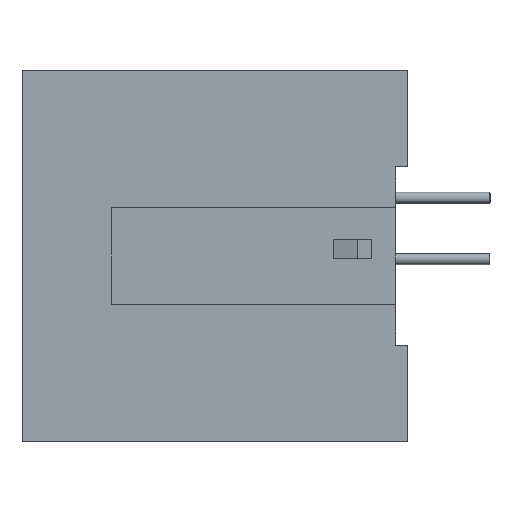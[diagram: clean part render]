
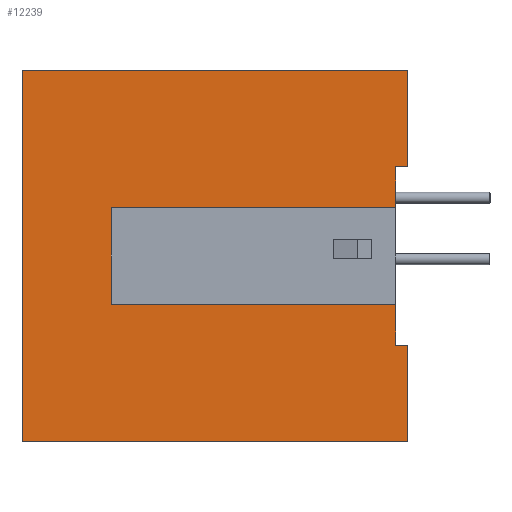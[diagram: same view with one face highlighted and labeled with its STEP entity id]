
A CAD part, left-side view. The second image highlights one B-rep face of the part: STEP entity #12239.
In plain terms, the highlighted planar face has unit normal (-1, 0, 0).
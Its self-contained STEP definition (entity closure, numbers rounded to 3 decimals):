
#409 = EDGE_CURVE ( 'NONE', #6827, #12593, #609, .T. ) ;
#457 = DIRECTION ( 'NONE',  ( 0., 0., 1. ) ) ;
#609 = LINE ( 'NONE', #684, #3271 ) ;
#684 = CARTESIAN_POINT ( 'NONE',  ( -27.5, 4., 0. ) ) ;
#745 = LINE ( 'NONE', #11575, #10384 ) ;
#837 = LINE ( 'NONE', #3326, #9380 ) ;
#955 = ORIENTED_EDGE ( 'NONE', *, *, #2630, .T. ) ;
#1096 = LINE ( 'NONE', #13087, #2777 ) ;
#1269 = CARTESIAN_POINT ( 'NONE',  ( -27.5, -8.3, 7.7 ) ) ;
#1413 = LINE ( 'NONE', #6178, #6186 ) ;
#1547 = LINE ( 'NONE', #4185, #4144 ) ;
#1643 = CARTESIAN_POINT ( 'NONE',  ( -27.5, -0.3, 1.8 ) ) ;
#1660 = VECTOR ( 'NONE', #3234, 1000. ) ;
#1877 = LINE ( 'NONE', #1643, #12169 ) ;
#2078 = ORIENTED_EDGE ( 'NONE', *, *, #5729, .F. ) ;
#2206 = CARTESIAN_POINT ( 'NONE',  ( -27.5, -7.8, 1.8 ) ) ;
#2349 = CARTESIAN_POINT ( 'NONE',  ( -27.5, 4., 1.8 ) ) ;
#2397 = VERTEX_POINT ( 'NONE', #2206 ) ;
#2450 = VERTEX_POINT ( 'NONE', #8057 ) ;
#2509 = CARTESIAN_POINT ( 'NONE',  ( -27.5, -8.3, -3.7 ) ) ;
#2519 = CARTESIAN_POINT ( 'NONE',  ( -27.5, -0.3, -7.7 ) ) ;
#2630 = EDGE_CURVE ( 'NONE', #14668, #4845, #1413, .T. ) ;
#2739 = ORIENTED_EDGE ( 'NONE', *, *, #7478, .F. ) ;
#2777 = VECTOR ( 'NONE', #5856, 1000. ) ;
#2883 = LINE ( 'NONE', #2519, #10856 ) ;
#3023 = VECTOR ( 'NONE', #14597, 1000. ) ;
#3026 = ORIENTED_EDGE ( 'NONE', *, *, #3966, .F. ) ;
#3234 = DIRECTION ( 'NONE',  ( 0., -1., 0. ) ) ;
#3271 = VECTOR ( 'NONE', #13538, 1000. ) ;
#3326 = CARTESIAN_POINT ( 'NONE',  ( -27.5, -0.3, 3.7 ) ) ;
#3514 = VECTOR ( 'NONE', #11791, 1000. ) ;
#3703 = VERTEX_POINT ( 'NONE', #2509 ) ;
#3966 = EDGE_CURVE ( 'NONE', #5069, #11071, #1096, .T. ) ;
#4144 = VECTOR ( 'NONE', #7702, 1000. ) ;
#4185 = CARTESIAN_POINT ( 'NONE',  ( -27.5, -0.3, -1.8 ) ) ;
#4594 = FACE_OUTER_BOUND ( 'NONE', #12394, .T. ) ;
#4845 = VERTEX_POINT ( 'NONE', #8165 ) ;
#5069 = VERTEX_POINT ( 'NONE', #12424 ) ;
#5098 = CARTESIAN_POINT ( 'NONE',  ( -27.5, -8.3, 0. ) ) ;
#5292 = EDGE_CURVE ( 'NONE', #2450, #14650, #2883, .T. ) ;
#5424 = CARTESIAN_POINT ( 'NONE',  ( -27.5, -0.3, -3.7 ) ) ;
#5729 = EDGE_CURVE ( 'NONE', #14650, #4845, #9967, .T. ) ;
#5740 = LINE ( 'NONE', #5424, #1660 ) ;
#5785 = PLANE ( 'NONE',  #6458 ) ;
#5856 = DIRECTION ( 'NONE',  ( 0., 0., -1. ) ) ;
#5911 = CARTESIAN_POINT ( 'NONE',  ( -27.5, 4., -1.8 ) ) ;
#6031 = LINE ( 'NONE', #8366, #3514 ) ;
#6178 = CARTESIAN_POINT ( 'NONE',  ( -27.5, -0.3, 7.7 ) ) ;
#6186 = VECTOR ( 'NONE', #10922, 1000. ) ;
#6231 = CARTESIAN_POINT ( 'NONE',  ( -27.5, 7.7, 0. ) ) ;
#6319 = VERTEX_POINT ( 'NONE', #12815 ) ;
#6458 = AXIS2_PLACEMENT_3D ( 'NONE', #8111, #12863, #11467 ) ;
#6827 = VERTEX_POINT ( 'NONE', #2349 ) ;
#7039 = ORIENTED_EDGE ( 'NONE', *, *, #7453, .F. ) ;
#7453 = EDGE_CURVE ( 'NONE', #11071, #3703, #5740, .T. ) ;
#7478 = EDGE_CURVE ( 'NONE', #14081, #2397, #745, .T. ) ;
#7582 = DIRECTION ( 'NONE',  ( 0., 1., 0. ) ) ;
#7702 = DIRECTION ( 'NONE',  ( 0., -1., 0. ) ) ;
#8057 = CARTESIAN_POINT ( 'NONE',  ( -27.5, -8.3, -7.7 ) ) ;
#8111 = CARTESIAN_POINT ( 'NONE',  ( -27.5, -8.62, -8.008 ) ) ;
#8165 = CARTESIAN_POINT ( 'NONE',  ( -27.5, 7.7, 7.7 ) ) ;
#8366 = CARTESIAN_POINT ( 'NONE',  ( -27.5, -8.3, 0. ) ) ;
#9072 = CARTESIAN_POINT ( 'NONE',  ( -27.5, -7.8, -3.7 ) ) ;
#9111 = ORIENTED_EDGE ( 'NONE', *, *, #409, .F. ) ;
#9242 = DIRECTION ( 'NONE',  ( 0., 0., -1. ) ) ;
#9380 = VECTOR ( 'NONE', #15015, 1000. ) ;
#9967 = LINE ( 'NONE', #6231, #10132 ) ;
#10132 = VECTOR ( 'NONE', #457, 1000. ) ;
#10136 = DIRECTION ( 'NONE',  ( 0., 1., 0. ) ) ;
#10384 = VECTOR ( 'NONE', #9242, 1000. ) ;
#10611 = ORIENTED_EDGE ( 'NONE', *, *, #12038, .F. ) ;
#10856 = VECTOR ( 'NONE', #10136, 1000. ) ;
#10922 = DIRECTION ( 'NONE',  ( 0., 1., 0. ) ) ;
#11071 = VERTEX_POINT ( 'NONE', #9072 ) ;
#11112 = EDGE_CURVE ( 'NONE', #3703, #2450, #6031, .T. ) ;
#11467 = DIRECTION ( 'NONE',  ( 0., 1., 0. ) ) ;
#11507 = EDGE_CURVE ( 'NONE', #14668, #6319, #12039, .T. ) ;
#11575 = CARTESIAN_POINT ( 'NONE',  ( -27.5, -7.8, 0. ) ) ;
#11587 = CARTESIAN_POINT ( 'NONE',  ( -27.5, -7.8, 3.7 ) ) ;
#11791 = DIRECTION ( 'NONE',  ( 0., 0., -1. ) ) ;
#12038 = EDGE_CURVE ( 'NONE', #2397, #6827, #1877, .T. ) ;
#12039 = LINE ( 'NONE', #5098, #3023 ) ;
#12169 = VECTOR ( 'NONE', #7582, 1000. ) ;
#12239 = ADVANCED_FACE ( 'NONE', ( #4594 ), #5785, .F. ) ;
#12394 = EDGE_LOOP ( 'NONE', ( #13360, #955, #2078, #14040, #13106, #7039, #3026, #14829, #9111, #10611, #2739, #15207 ) ) ;
#12424 = CARTESIAN_POINT ( 'NONE',  ( -27.5, -7.8, -1.8 ) ) ;
#12593 = VERTEX_POINT ( 'NONE', #5911 ) ;
#12815 = CARTESIAN_POINT ( 'NONE',  ( -27.5, -8.3, 3.7 ) ) ;
#12863 = DIRECTION ( 'NONE',  ( 1., 0., 0. ) ) ;
#13031 = CARTESIAN_POINT ( 'NONE',  ( -27.5, 7.7, -7.7 ) ) ;
#13087 = CARTESIAN_POINT ( 'NONE',  ( -27.5, -7.8, 0. ) ) ;
#13106 = ORIENTED_EDGE ( 'NONE', *, *, #11112, .F. ) ;
#13360 = ORIENTED_EDGE ( 'NONE', *, *, #11507, .F. ) ;
#13538 = DIRECTION ( 'NONE',  ( 0., 0., -1. ) ) ;
#14014 = EDGE_CURVE ( 'NONE', #12593, #5069, #1547, .T. ) ;
#14040 = ORIENTED_EDGE ( 'NONE', *, *, #5292, .F. ) ;
#14081 = VERTEX_POINT ( 'NONE', #11587 ) ;
#14126 = EDGE_CURVE ( 'NONE', #6319, #14081, #837, .T. ) ;
#14597 = DIRECTION ( 'NONE',  ( 0., 0., -1. ) ) ;
#14650 = VERTEX_POINT ( 'NONE', #13031 ) ;
#14668 = VERTEX_POINT ( 'NONE', #1269 ) ;
#14829 = ORIENTED_EDGE ( 'NONE', *, *, #14014, .F. ) ;
#15015 = DIRECTION ( 'NONE',  ( 0., 1., 0. ) ) ;
#15207 = ORIENTED_EDGE ( 'NONE', *, *, #14126, .F. ) ;
